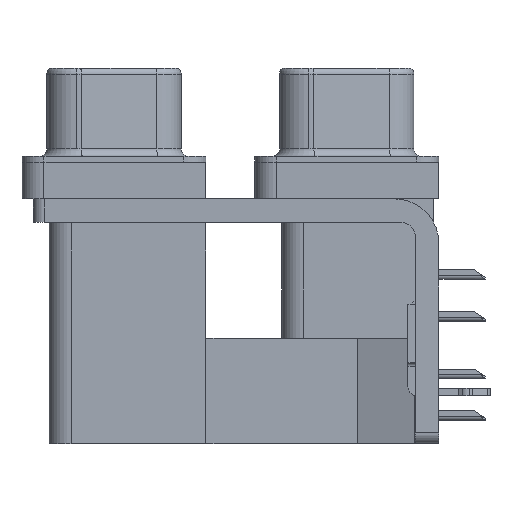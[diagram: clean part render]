
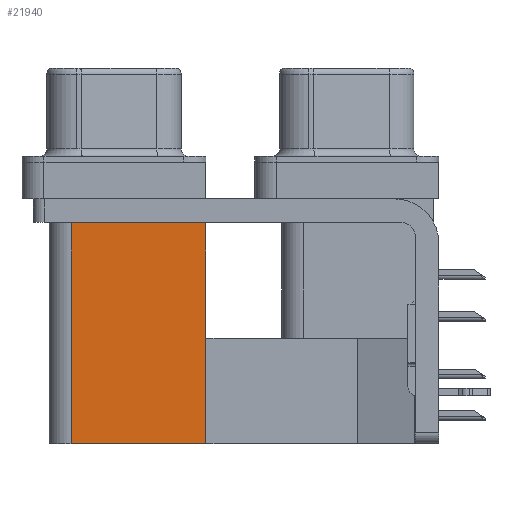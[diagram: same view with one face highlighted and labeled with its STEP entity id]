
A CAD part, left-side view. The second image highlights one B-rep face of the part: STEP entity #21940.
In plain terms, the highlighted planar face has unit normal (-1, 0, 0).
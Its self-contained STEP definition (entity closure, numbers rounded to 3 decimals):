
#100 = AXIS2_PLACEMENT_3D ( 'NONE', #3058, #19855, #7257 ) ;
#1593 = CARTESIAN_POINT ( 'NONE',  ( 3.79, 9.6, -2.5 ) ) ;
#1728 = EDGE_CURVE ( 'NONE', #4488, #17261, #4136, .T. ) ;
#1835 = VECTOR ( 'NONE', #26151, 1000. ) ;
#3007 = ORIENTED_EDGE ( 'NONE', *, *, #18794, .F. ) ;
#3058 = CARTESIAN_POINT ( 'NONE',  ( 3.79, 9.6, -19.2 ) ) ;
#3646 = EDGE_CURVE ( 'NONE', #17261, #24176, #14310, .T. ) ;
#4136 = LINE ( 'NONE', #12105, #11467 ) ;
#4467 = VECTOR ( 'NONE', #5813, 1000. ) ;
#4488 = VERTEX_POINT ( 'NONE', #26166 ) ;
#4489 = VERTEX_POINT ( 'NONE', #22000 ) ;
#5352 = VECTOR ( 'NONE', #26301, 1000. ) ;
#5406 = ORIENTED_EDGE ( 'NONE', *, *, #1728, .T. ) ;
#5813 = DIRECTION ( 'NONE',  ( 0., 1., 0. ) ) ;
#6600 = LINE ( 'NONE', #17770, #5352 ) ;
#7257 = DIRECTION ( 'NONE',  ( 0., 0., -1. ) ) ;
#8066 = ORIENTED_EDGE ( 'NONE', *, *, #3646, .T. ) ;
#9979 = CARTESIAN_POINT ( 'NONE',  ( 3.79, 9.6, -2.5 ) ) ;
#10422 = DIRECTION ( 'NONE',  ( 0., 0., 1. ) ) ;
#11464 = LINE ( 'NONE', #22257, #1835 ) ;
#11467 = VECTOR ( 'NONE', #10422, 1000. ) ;
#12105 = CARTESIAN_POINT ( 'NONE',  ( 3.79, 9.6, -19.2 ) ) ;
#12239 = EDGE_CURVE ( 'NONE', #4488, #4489, #11464, .T. ) ;
#13137 = ORIENTED_EDGE ( 'NONE', *, *, #12239, .F. ) ;
#13337 = CARTESIAN_POINT ( 'NONE',  ( 3.79, 18.8, -2.5 ) ) ;
#14310 = LINE ( 'NONE', #9979, #4467 ) ;
#17261 = VERTEX_POINT ( 'NONE', #1593 ) ;
#17418 = EDGE_LOOP ( 'NONE', ( #8066, #3007, #13137, #5406 ) ) ;
#17770 = CARTESIAN_POINT ( 'NONE',  ( 3.79, 18.8, -19.2 ) ) ;
#18794 = EDGE_CURVE ( 'NONE', #4489, #24176, #6600, .T. ) ;
#19855 = DIRECTION ( 'NONE',  ( 1., 0., 0. ) ) ;
#21940 = ADVANCED_FACE ( 'NONE', ( #26528 ), #24300, .F. ) ;
#22000 = CARTESIAN_POINT ( 'NONE',  ( 3.79, 18.8, -19.2 ) ) ;
#22257 = CARTESIAN_POINT ( 'NONE',  ( 3.79, 9.6, -19.2 ) ) ;
#24176 = VERTEX_POINT ( 'NONE', #13337 ) ;
#24300 = PLANE ( 'NONE',  #100 ) ;
#26151 = DIRECTION ( 'NONE',  ( 0., 1., 0. ) ) ;
#26166 = CARTESIAN_POINT ( 'NONE',  ( 3.79, 9.6, -19.2 ) ) ;
#26301 = DIRECTION ( 'NONE',  ( 0., 0., 1. ) ) ;
#26528 = FACE_OUTER_BOUND ( 'NONE', #17418, .T. ) ;
